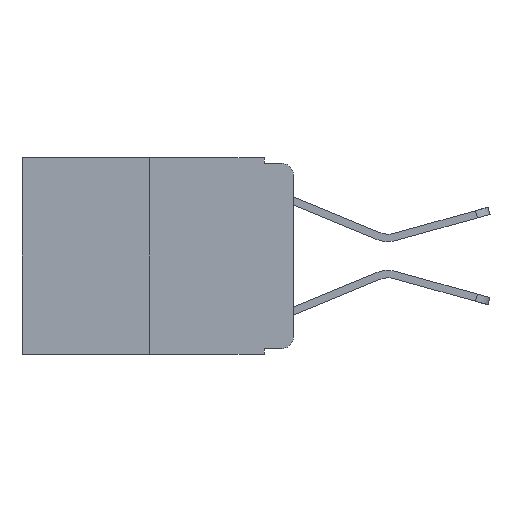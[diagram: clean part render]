
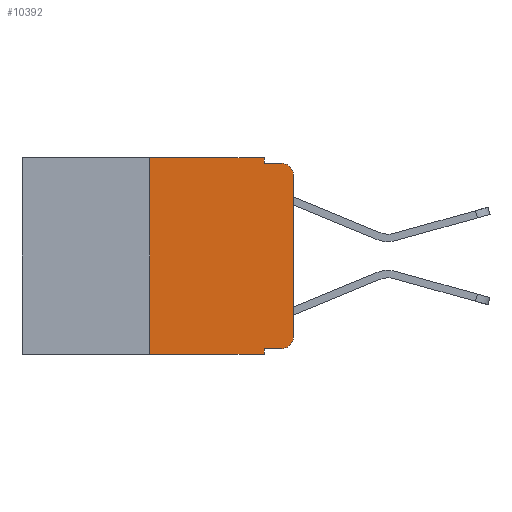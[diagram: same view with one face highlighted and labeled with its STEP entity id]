
A CAD part, left-side view. The second image highlights one B-rep face of the part: STEP entity #10392.
In plain terms, the highlighted planar face has unit normal (-1, 0, 0).
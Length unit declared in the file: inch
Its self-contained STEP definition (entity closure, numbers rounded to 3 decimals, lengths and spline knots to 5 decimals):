
#11 = CARTESIAN_POINT ( 'NONE',  ( 0., 0.051, -0.01 ) ) ;
#77 = CARTESIAN_POINT ( 'NONE',  ( 0., 0.473, -0.343 ) ) ;
#97 = CARTESIAN_POINT ( 'NONE',  ( 0., 0.051, 0. ) ) ;
#142 = ORIENTED_EDGE ( 'NONE', *, *, #2095, .F. ) ;
#276 = DIRECTION ( 'NONE',  ( -1., 0., 0. ) ) ;
#495 = CARTESIAN_POINT ( 'NONE',  ( 0., 0.051, -0.343 ) ) ;
#525 = VERTEX_POINT ( 'NONE', #1893 ) ;
#695 = EDGE_LOOP ( 'NONE', ( #4318, #8829, #4605, #142, #7385, #9621, #9886, #5675, #10432, #1516 ) ) ;
#697 = VERTEX_POINT ( 'NONE', #6879 ) ;
#838 = LINE ( 'NONE', #4229, #10038 ) ;
#874 = LINE ( 'NONE', #77, #5046 ) ;
#918 = EDGE_CURVE ( 'NONE', #6560, #1428, #5622, .T. ) ;
#1013 = DIRECTION ( 'NONE',  ( 1., 0., 0. ) ) ;
#1048 = AXIS2_PLACEMENT_3D ( 'NONE', #6262, #1013, #7137 ) ;
#1292 = CARTESIAN_POINT ( 'NONE',  ( 0., 0.25, 0. ) ) ;
#1383 = VERTEX_POINT ( 'NONE', #9020 ) ;
#1428 = VERTEX_POINT ( 'NONE', #1292 ) ;
#1516 = ORIENTED_EDGE ( 'NONE', *, *, #4732, .T. ) ;
#1535 = DIRECTION ( 'NONE',  ( 0., 0., 1. ) ) ;
#1545 = LINE ( 'NONE', #9222, #5448 ) ;
#1698 = DIRECTION ( 'NONE',  ( 0., 0., -1. ) ) ;
#1839 = DIRECTION ( 'NONE',  ( 0., -1., 0. ) ) ;
#1893 = CARTESIAN_POINT ( 'NONE',  ( 0., 0., -0.03 ) ) ;
#2095 = EDGE_CURVE ( 'NONE', #697, #10333, #3824, .T. ) ;
#2418 = CARTESIAN_POINT ( 'NONE',  ( 0., 0.051, -0.333 ) ) ;
#2549 = VERTEX_POINT ( 'NONE', #5346 ) ;
#2811 = AXIS2_PLACEMENT_3D ( 'NONE', #9726, #276, #1698 ) ;
#3311 = EDGE_CURVE ( 'NONE', #1428, #697, #1545, .T. ) ;
#3479 = CIRCLE ( 'NONE', #2811, 0.02 ) ;
#3622 = LINE ( 'NONE', #6380, #7896 ) ;
#3824 = LINE ( 'NONE', #10067, #4104 ) ;
#3905 = DIRECTION ( 'NONE',  ( -1., 0., 0. ) ) ;
#4104 = VECTOR ( 'NONE', #9903, 39.37008 ) ;
#4229 = CARTESIAN_POINT ( 'NONE',  ( 0., 0., 0. ) ) ;
#4318 = ORIENTED_EDGE ( 'NONE', *, *, #9614, .T. ) ;
#4370 = VECTOR ( 'NONE', #6268, 39.37008 ) ;
#4524 = EDGE_CURVE ( 'NONE', #10333, #1383, #3622, .T. ) ;
#4605 = ORIENTED_EDGE ( 'NONE', *, *, #4524, .F. ) ;
#4622 = VERTEX_POINT ( 'NONE', #495 ) ;
#4732 = EDGE_CURVE ( 'NONE', #9493, #2549, #3479, .T. ) ;
#4837 = AXIS2_PLACEMENT_3D ( 'NONE', #8992, #3905, #9847 ) ;
#5046 = VECTOR ( 'NONE', #1839, 39.37008 ) ;
#5346 = CARTESIAN_POINT ( 'NONE',  ( 0., 0., -0.313 ) ) ;
#5448 = VECTOR ( 'NONE', #10668, 39.37008 ) ;
#5622 = LINE ( 'NONE', #10972, #10382 ) ;
#5675 = ORIENTED_EDGE ( 'NONE', *, *, #9820, .F. ) ;
#6262 = CARTESIAN_POINT ( 'NONE',  ( 0., 0.473, 0. ) ) ;
#6268 = DIRECTION ( 'NONE',  ( 0., 0., -1. ) ) ;
#6380 = CARTESIAN_POINT ( 'NONE',  ( 0., 0.051, -0.01 ) ) ;
#6560 = VERTEX_POINT ( 'NONE', #8144 ) ;
#6663 = DIRECTION ( 'NONE',  ( 0., -1., 0. ) ) ;
#6850 = CARTESIAN_POINT ( 'NONE',  ( 0., 0.051, -0.333 ) ) ;
#6879 = CARTESIAN_POINT ( 'NONE',  ( 0., 0.051, 0. ) ) ;
#7053 = CIRCLE ( 'NONE', #4837, 0.02 ) ;
#7137 = DIRECTION ( 'NONE',  ( 0., 0., -1. ) ) ;
#7385 = ORIENTED_EDGE ( 'NONE', *, *, #3311, .F. ) ;
#7605 = DIRECTION ( 'NONE',  ( 0., -1., 0. ) ) ;
#7815 = FACE_OUTER_BOUND ( 'NONE', #695, .T. ) ;
#7896 = VECTOR ( 'NONE', #6663, 39.37008 ) ;
#7919 = EDGE_CURVE ( 'NONE', #525, #1383, #7053, .T. ) ;
#8141 = EDGE_CURVE ( 'NONE', #8818, #9493, #9673, .T. ) ;
#8144 = CARTESIAN_POINT ( 'NONE',  ( 0., 0.25, -0.343 ) ) ;
#8326 = CARTESIAN_POINT ( 'NONE',  ( 0., 0.02, -0.333 ) ) ;
#8358 = EDGE_CURVE ( 'NONE', #6560, #4622, #874, .T. ) ;
#8818 = VERTEX_POINT ( 'NONE', #6850 ) ;
#8829 = ORIENTED_EDGE ( 'NONE', *, *, #7919, .T. ) ;
#8992 = CARTESIAN_POINT ( 'NONE',  ( 0., 0.02, -0.03 ) ) ;
#9020 = CARTESIAN_POINT ( 'NONE',  ( 0., 0.02, -0.01 ) ) ;
#9222 = CARTESIAN_POINT ( 'NONE',  ( 0., 0.473, 0. ) ) ;
#9308 = DIRECTION ( 'NONE',  ( 0., 0., 1. ) ) ;
#9411 = VECTOR ( 'NONE', #7605, 39.37008 ) ;
#9493 = VERTEX_POINT ( 'NONE', #8326 ) ;
#9614 = EDGE_CURVE ( 'NONE', #2549, #525, #838, .T. ) ;
#9621 = ORIENTED_EDGE ( 'NONE', *, *, #918, .F. ) ;
#9673 = LINE ( 'NONE', #2418, #9411 ) ;
#9726 = CARTESIAN_POINT ( 'NONE',  ( 0., 0.02, -0.313 ) ) ;
#9820 = EDGE_CURVE ( 'NONE', #8818, #4622, #10865, .T. ) ;
#9847 = DIRECTION ( 'NONE',  ( 0., 0., -1. ) ) ;
#9886 = ORIENTED_EDGE ( 'NONE', *, *, #8358, .T. ) ;
#9903 = DIRECTION ( 'NONE',  ( 0., 0., -1. ) ) ;
#10038 = VECTOR ( 'NONE', #9308, 39.37008 ) ;
#10067 = CARTESIAN_POINT ( 'NONE',  ( 0., 0.051, 0. ) ) ;
#10333 = VERTEX_POINT ( 'NONE', #11 ) ;
#10382 = VECTOR ( 'NONE', #1535, 39.37008 ) ;
#10392 = ADVANCED_FACE ( 'NONE', ( #7815 ), #10500, .F. ) ;
#10432 = ORIENTED_EDGE ( 'NONE', *, *, #8141, .T. ) ;
#10500 = PLANE ( 'NONE',  #1048 ) ;
#10668 = DIRECTION ( 'NONE',  ( 0., -1., 0. ) ) ;
#10865 = LINE ( 'NONE', #97, #4370 ) ;
#10972 = CARTESIAN_POINT ( 'NONE',  ( 0., 0.25, 0. ) ) ;
